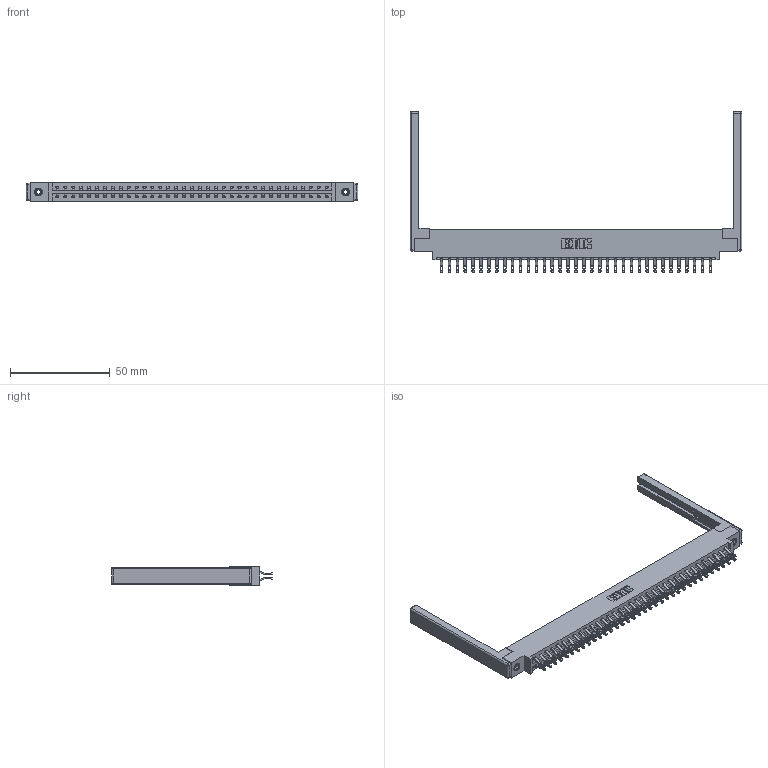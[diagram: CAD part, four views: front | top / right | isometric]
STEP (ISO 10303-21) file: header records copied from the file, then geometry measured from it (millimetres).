
FILE_DESCRIPTION (( 'STEP AP203' ), '1' );
FILE_NAME ('387-070-555-868.STEP', '2019-10-21T22:54:44', ( '' ), ( '' ), 'SwSTEP 2.0', 'SolidWorks 2016', '' );
FILE_SCHEMA (( 'CONFIG_CONTROL_DESIGN' ));
Length unit declared in the file: inch
Products named in the file (5): 345-250-001_345-250-001-102; 387-070-555-868; 307-220-068; 337 Part_0.170 Offset - 0.156 Dia-TI; 345-292-001_555 Tail
Assembly tree (75 placements, depth 2):
  387-070-555-868
    337 Part_0.170 Offset - 0.156 Dia-TI
    345-292-001_555 Tail  x70
    345-250-001_345-250-001-102  x2
    307-220-068  x2
Bounding box: 166.12 x 80.52 x 9.4 mm (x, y, z)
Volume: 21883.8 mm3; surface area: 24622 mm2
Topology: 75 solids, 75 shells, 4472 faces, 13943 edges, 9274 vertices
Faces by surface type: plane 2682, cylinder 1766, cone 12, sphere 8, torus 4
Entity records: 31260 total; most frequent: CARTESIAN_POINT 5273, ORIENTED_EDGE 5168, DIRECTION 4538, EDGE_CURVE 2584, VECTOR 2386, LINE 2386, VERTEX_POINT 1714, AXIS2_PLACEMENT_3D 1076
